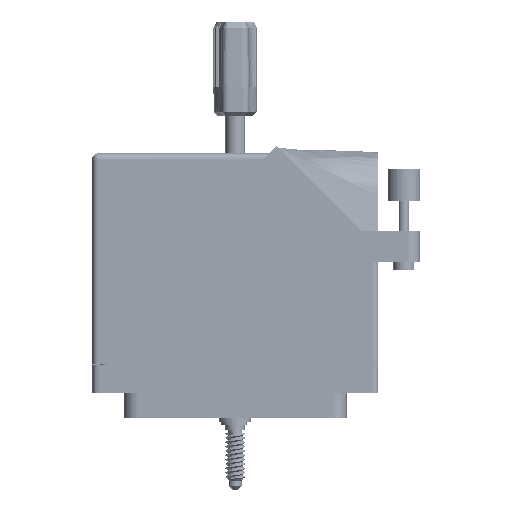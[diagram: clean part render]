
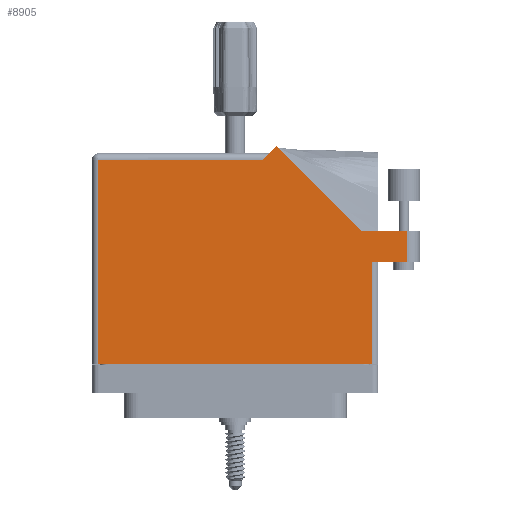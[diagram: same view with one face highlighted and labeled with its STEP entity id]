
A CAD part, front view. The second image highlights one B-rep face of the part: STEP entity #8905.
In plain terms, the highlighted face is planar.
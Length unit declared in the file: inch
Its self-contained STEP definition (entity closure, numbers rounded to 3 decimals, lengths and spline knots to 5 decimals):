
#495 = FACE_OUTER_BOUND ( 'NONE', #40073, .T. ) ;
#3344 = LINE ( 'NONE', #27154, #87693 ) ;
#5064 = CARTESIAN_POINT ( 'NONE',  ( 1.6525, 0.88, 0.765 ) ) ;
#5319 = VERTEX_POINT ( 'NONE', #5064 ) ;
#8905 = ADVANCED_FACE ( 'NONE', ( #495 ), #87650, .F. ) ;
#12299 = LINE ( 'NONE', #37474, #23793 ) ;
#14070 = DIRECTION ( 'NONE',  ( 1., 0., 0. ) ) ;
#15904 = LINE ( 'NONE', #95168, #83653 ) ;
#16401 = LINE ( 'NONE', #82168, #100690 ) ;
#16673 = VERTEX_POINT ( 'NONE', #88617 ) ;
#21326 = VERTEX_POINT ( 'NONE', #64228 ) ;
#23793 = VECTOR ( 'NONE', #45321, 39.37008 ) ;
#24671 = ORIENTED_EDGE ( 'NONE', *, *, #60810, .T. ) ;
#25895 = DIRECTION ( 'NONE',  ( 0., 1., 0. ) ) ;
#26806 = DIRECTION ( 'NONE',  ( 0., -1., 0. ) ) ;
#27154 = CARTESIAN_POINT ( 'NONE',  ( -1.3155, -0.1, 0.765 ) ) ;
#27726 = LINE ( 'NONE', #31788, #57147 ) ;
#28359 = CARTESIAN_POINT ( 'NONE',  ( 0.39821, 2.00071, 0.765 ) ) ;
#28512 = DIRECTION ( 'NONE',  ( 1., 0., 0. ) ) ;
#28797 = DIRECTION ( 'NONE',  ( 0., 1., 0. ) ) ;
#30529 = DIRECTION ( 'NONE',  ( 0., 0., -1. ) ) ;
#31788 = CARTESIAN_POINT ( 'NONE',  ( 1.7775, 1.187, 0.765 ) ) ;
#31911 = CARTESIAN_POINT ( 'NONE',  ( -1.3775, -0.1, 0.765 ) ) ;
#32144 = DIRECTION ( 'NONE',  ( -1., 0., 0. ) ) ;
#32930 = EDGE_CURVE ( 'NONE', #21326, #16673, #27726, .T. ) ;
#35062 = CARTESIAN_POINT ( 'NONE',  ( 0.2655, 1.868, 0.765 ) ) ;
#35802 = CARTESIAN_POINT ( 'NONE',  ( 1.3155, -0.1, 0.765 ) ) ;
#36154 = LINE ( 'NONE', #101303, #56588 ) ;
#37474 = CARTESIAN_POINT ( 'NONE',  ( 1.21192, 1.187, 0.765 ) ) ;
#40073 = EDGE_LOOP ( 'NONE', ( #42405, #85104, #58559, #24671, #86688, #44899, #46665, #92720, #48769 ) ) ;
#42405 = ORIENTED_EDGE ( 'NONE', *, *, #102276, .T. ) ;
#42529 = VECTOR ( 'NONE', #81014, 39.37008 ) ;
#44899 = ORIENTED_EDGE ( 'NONE', *, *, #78967, .T. ) ;
#45321 = DIRECTION ( 'NONE',  ( -0.707, 0.707, 0. ) ) ;
#46665 = ORIENTED_EDGE ( 'NONE', *, *, #60635, .T. ) ;
#47280 = CARTESIAN_POINT ( 'NONE',  ( -1.3775, 1.93, 0.765 ) ) ;
#48769 = ORIENTED_EDGE ( 'NONE', *, *, #68940, .T. ) ;
#49524 = CARTESIAN_POINT ( 'NONE',  ( -1.3155, 1.868, 0.765 ) ) ;
#51355 = LINE ( 'NONE', #68013, #75638 ) ;
#51488 = VERTEX_POINT ( 'NONE', #28359 ) ;
#56588 = VECTOR ( 'NONE', #28512, 39.37008 ) ;
#57147 = VECTOR ( 'NONE', #32144, 39.37008 ) ;
#58559 = ORIENTED_EDGE ( 'NONE', *, *, #32930, .T. ) ;
#59080 = CARTESIAN_POINT ( 'NONE',  ( 1.3155, 0.88, 0.765 ) ) ;
#60635 = EDGE_CURVE ( 'NONE', #98942, #89175, #3344, .T. ) ;
#60810 = EDGE_CURVE ( 'NONE', #16673, #51488, #12299, .T. ) ;
#63802 = VECTOR ( 'NONE', #14070, 39.37008 ) ;
#64228 = CARTESIAN_POINT ( 'NONE',  ( 1.6525, 1.187, 0.765 ) ) ;
#64262 = LINE ( 'NONE', #102549, #42529 ) ;
#64659 = DIRECTION ( 'NONE',  ( -0.707, -0.707, 0. ) ) ;
#68013 = CARTESIAN_POINT ( 'NONE',  ( 1.3155, 0.88, 0.765 ) ) ;
#68874 = VERTEX_POINT ( 'NONE', #59080 ) ;
#68940 = EDGE_CURVE ( 'NONE', #91644, #68874, #51355, .T. ) ;
#74227 = CARTESIAN_POINT ( 'NONE',  ( -1.3155, -0.1, 0.765 ) ) ;
#75638 = VECTOR ( 'NONE', #25895, 39.37008 ) ;
#76115 = EDGE_CURVE ( 'NONE', #51488, #77836, #16401, .T. ) ;
#77836 = VERTEX_POINT ( 'NONE', #35062 ) ;
#78967 = EDGE_CURVE ( 'NONE', #77836, #98942, #64262, .T. ) ;
#81014 = DIRECTION ( 'NONE',  ( -1., 0., 0. ) ) ;
#82168 = CARTESIAN_POINT ( 'NONE',  ( 0.3275, 1.93, 0.765 ) ) ;
#83653 = VECTOR ( 'NONE', #28797, 39.37008 ) ;
#85104 = ORIENTED_EDGE ( 'NONE', *, *, #101129, .T. ) ;
#85546 = LINE ( 'NONE', #31911, #63802 ) ;
#86688 = ORIENTED_EDGE ( 'NONE', *, *, #76115, .T. ) ;
#87650 = PLANE ( 'NONE',  #95505 ) ;
#87693 = VECTOR ( 'NONE', #26806, 39.37008 ) ;
#88617 = CARTESIAN_POINT ( 'NONE',  ( 1.21192, 1.187, 0.765 ) ) ;
#89175 = VERTEX_POINT ( 'NONE', #74227 ) ;
#91263 = EDGE_CURVE ( 'NONE', #89175, #91644, #85546, .T. ) ;
#91644 = VERTEX_POINT ( 'NONE', #35802 ) ;
#92720 = ORIENTED_EDGE ( 'NONE', *, *, #91263, .T. ) ;
#95168 = CARTESIAN_POINT ( 'NONE',  ( 1.6525, 1.187, 0.765 ) ) ;
#95505 = AXIS2_PLACEMENT_3D ( 'NONE', #47280, #30529, #95849 ) ;
#95849 = DIRECTION ( 'NONE',  ( -1., 0., 0. ) ) ;
#98942 = VERTEX_POINT ( 'NONE', #49524 ) ;
#100690 = VECTOR ( 'NONE', #64659, 39.37008 ) ;
#101129 = EDGE_CURVE ( 'NONE', #5319, #21326, #15904, .T. ) ;
#101303 = CARTESIAN_POINT ( 'NONE',  ( 1.3775, 0.88, 0.765 ) ) ;
#102276 = EDGE_CURVE ( 'NONE', #68874, #5319, #36154, .T. ) ;
#102549 = CARTESIAN_POINT ( 'NONE',  ( -1.3775, 1.868, 0.765 ) ) ;
